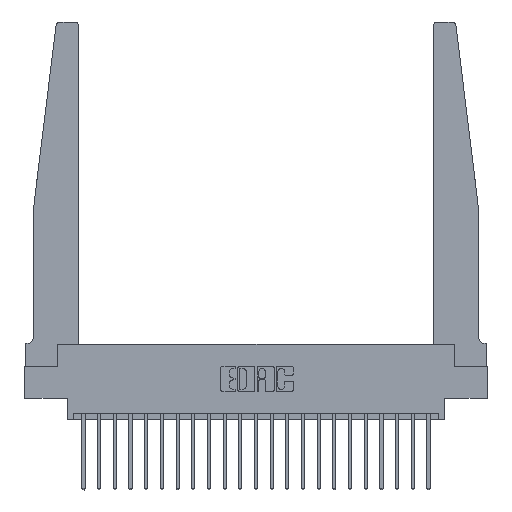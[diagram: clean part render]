
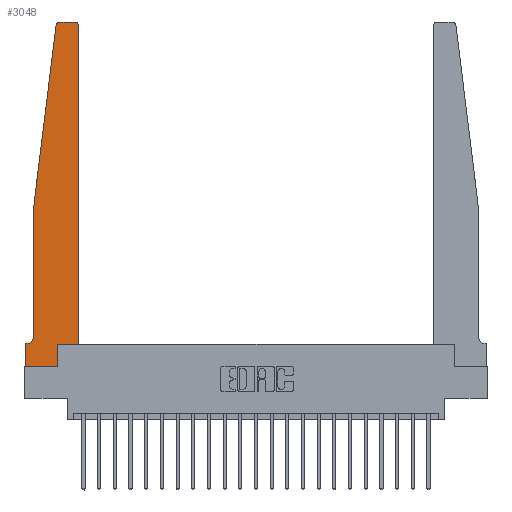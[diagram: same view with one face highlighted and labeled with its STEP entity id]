
A CAD part, top view. The second image highlights one B-rep face of the part: STEP entity #3048.
In plain terms, the highlighted planar face has unit normal (0, 0, 1).
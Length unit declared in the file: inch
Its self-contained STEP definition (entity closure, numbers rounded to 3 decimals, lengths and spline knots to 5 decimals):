
#40 = CARTESIAN_POINT ( 'NONE',  ( 0., 0.1875, 0.37 ) ) ;
#45 = CARTESIAN_POINT ( 'NONE',  ( 0., 0., 0.37 ) ) ;
#124 = EDGE_CURVE ( 'NONE', #2681, #18343, #1156, .T. ) ;
#596 = VECTOR ( 'NONE', #16283, 39.37008 ) ;
#807 = CARTESIAN_POINT ( 'NONE',  ( 0.425, 0.18, 0.37 ) ) ;
#1056 = CARTESIAN_POINT ( 'NONE',  ( 0.015, 0.2375, 0.37 ) ) ;
#1156 = LINE ( 'NONE', #21388, #596 ) ;
#1567 = AXIS2_PLACEMENT_3D ( 'NONE', #7672, #19767, #9418 ) ;
#1775 = CARTESIAN_POINT ( 'NONE',  ( 0.425, 0.18, 0.37 ) ) ;
#1826 = DIRECTION ( 'NONE',  ( 1., 0., 0. ) ) ;
#1832 = DIRECTION ( 'NONE',  ( 0., -1., 0. ) ) ;
#2221 = CARTESIAN_POINT ( 'NONE',  ( 0.24675, 2.72367, 0.37 ) ) ;
#2587 = VERTEX_POINT ( 'NONE', #7590 ) ;
#2681 = VERTEX_POINT ( 'NONE', #16542 ) ;
#2718 = LINE ( 'NONE', #1775, #20107 ) ;
#2743 = LINE ( 'NONE', #8662, #16095 ) ;
#2776 = VERTEX_POINT ( 'NONE', #20132 ) ;
#2807 = DIRECTION ( 'NONE',  ( -1., 0., 0. ) ) ;
#3048 = ADVANCED_FACE ( 'NONE', ( #13934 ), #20865, .T. ) ;
#3137 = LINE ( 'NONE', #6098, #7814 ) ;
#3323 = AXIS2_PLACEMENT_3D ( 'NONE', #40, #12265, #1826 ) ;
#3652 = EDGE_LOOP ( 'NONE', ( #15649, #20769, #12135, #21859, #3939, #18905, #20501, #7257, #21600, #13485, #5334, #9979 ) ) ;
#3723 = VERTEX_POINT ( 'NONE', #5247 ) ;
#3742 = CARTESIAN_POINT ( 'NONE',  ( 0.065, 1.25, 0.37 ) ) ;
#3843 = LINE ( 'NONE', #7886, #7979 ) ;
#3939 = ORIENTED_EDGE ( 'NONE', *, *, #8789, .T. ) ;
#4183 = EDGE_CURVE ( 'NONE', #18343, #2776, #2743, .T. ) ;
#4529 = CARTESIAN_POINT ( 'NONE',  ( 0.395, 2.75, 0.37 ) ) ;
#4591 = AXIS2_PLACEMENT_3D ( 'NONE', #1056, #13247, #2807 ) ;
#4999 = DIRECTION ( 'NONE',  ( 0., -1., 0. ) ) ;
#5247 = CARTESIAN_POINT ( 'NONE',  ( 0., 0.1875, 0.37 ) ) ;
#5334 = ORIENTED_EDGE ( 'NONE', *, *, #10177, .T. ) ;
#5709 = EDGE_CURVE ( 'NONE', #22224, #11923, #6277, .T. ) ;
#6098 = CARTESIAN_POINT ( 'NONE',  ( 0.065, 0.1875, 0.37 ) ) ;
#6116 = DIRECTION ( 'NONE',  ( 1., 0., 0. ) ) ;
#6268 = CARTESIAN_POINT ( 'NONE',  ( 0.27653, 2.75, 0.37 ) ) ;
#6277 = LINE ( 'NONE', #3742, #16024 ) ;
#7116 = LINE ( 'NONE', #45, #15779 ) ;
#7257 = ORIENTED_EDGE ( 'NONE', *, *, #124, .T. ) ;
#7590 = CARTESIAN_POINT ( 'NONE',  ( 0.425, 2.72, 0.37 ) ) ;
#7672 = CARTESIAN_POINT ( 'NONE',  ( 0.27653, 2.72, 0.37 ) ) ;
#7814 = VECTOR ( 'NONE', #14745, 39.37008 ) ;
#7886 = CARTESIAN_POINT ( 'NONE',  ( 0.25, 2.75, 0.37 ) ) ;
#7979 = VECTOR ( 'NONE', #9639, 39.37008 ) ;
#8292 = EDGE_CURVE ( 'NONE', #11923, #20949, #19123, .T. ) ;
#8516 = CARTESIAN_POINT ( 'NONE',  ( 0.065, 1.25, 0.37 ) ) ;
#8662 = CARTESIAN_POINT ( 'NONE',  ( 0.2605, 0.18, 0.37 ) ) ;
#8789 = EDGE_CURVE ( 'NONE', #20949, #18746, #19098, .T. ) ;
#8946 = EDGE_CURVE ( 'NONE', #2587, #12451, #20955, .T. ) ;
#9377 = VECTOR ( 'NONE', #4999, 39.37008 ) ;
#9418 = DIRECTION ( 'NONE',  ( 1., 0., 0. ) ) ;
#9639 = DIRECTION ( 'NONE',  ( -1., 0., 0. ) ) ;
#9979 = ORIENTED_EDGE ( 'NONE', *, *, #8946, .T. ) ;
#10177 = EDGE_CURVE ( 'NONE', #18912, #2587, #2718, .T. ) ;
#10218 = CARTESIAN_POINT ( 'NONE',  ( 0.395, 2.72, 0.37 ) ) ;
#10550 = CARTESIAN_POINT ( 'NONE',  ( 0.015, 0.1875, 0.37 ) ) ;
#11923 = VERTEX_POINT ( 'NONE', #8516 ) ;
#11967 = DIRECTION ( 'NONE',  ( 1., 0., 0. ) ) ;
#12135 = ORIENTED_EDGE ( 'NONE', *, *, #5709, .T. ) ;
#12227 = DIRECTION ( 'NONE',  ( 0., 1., 0. ) ) ;
#12265 = DIRECTION ( 'NONE',  ( 0., 0., 1. ) ) ;
#12451 = VERTEX_POINT ( 'NONE', #4529 ) ;
#12926 = EDGE_CURVE ( 'NONE', #2776, #18912, #21606, .T. ) ;
#13247 = DIRECTION ( 'NONE',  ( 0., 0., -1. ) ) ;
#13485 = ORIENTED_EDGE ( 'NONE', *, *, #12926, .T. ) ;
#13730 = EDGE_CURVE ( 'NONE', #18746, #3723, #3137, .T. ) ;
#13934 = FACE_OUTER_BOUND ( 'NONE', #3652, .T. ) ;
#14374 = EDGE_CURVE ( 'NONE', #21360, #22224, #19311, .T. ) ;
#14745 = DIRECTION ( 'NONE',  ( -1., 0., 0. ) ) ;
#14801 = EDGE_CURVE ( 'NONE', #3723, #2681, #7116, .T. ) ;
#15066 = AXIS2_PLACEMENT_3D ( 'NONE', #10218, #22307, #11967 ) ;
#15649 = ORIENTED_EDGE ( 'NONE', *, *, #20711, .T. ) ;
#15779 = VECTOR ( 'NONE', #1832, 39.37008 ) ;
#16024 = VECTOR ( 'NONE', #17665, 39.37008 ) ;
#16095 = VECTOR ( 'NONE', #19024, 39.37008 ) ;
#16161 = CARTESIAN_POINT ( 'NONE',  ( 0.425, 0.18, 0.37 ) ) ;
#16283 = DIRECTION ( 'NONE',  ( 1., 0., 0. ) ) ;
#16497 = VECTOR ( 'NONE', #6116, 39.37008 ) ;
#16542 = CARTESIAN_POINT ( 'NONE',  ( 0., 0., 0.37 ) ) ;
#17051 = CARTESIAN_POINT ( 'NONE',  ( 0.065, 0.2375, 0.37 ) ) ;
#17149 = CARTESIAN_POINT ( 'NONE',  ( 0.065, 1.25, 0.37 ) ) ;
#17665 = DIRECTION ( 'NONE',  ( -0.122, -0.992, 0. ) ) ;
#17777 = CARTESIAN_POINT ( 'NONE',  ( 0.2605, 0., 0.37 ) ) ;
#18343 = VERTEX_POINT ( 'NONE', #17777 ) ;
#18746 = VERTEX_POINT ( 'NONE', #10550 ) ;
#18905 = ORIENTED_EDGE ( 'NONE', *, *, #13730, .T. ) ;
#18912 = VERTEX_POINT ( 'NONE', #16161 ) ;
#19024 = DIRECTION ( 'NONE',  ( 0., 1., 0. ) ) ;
#19098 = CIRCLE ( 'NONE', #4591, 0.05 ) ;
#19123 = LINE ( 'NONE', #17149, #9377 ) ;
#19311 = CIRCLE ( 'NONE', #1567, 0.03 ) ;
#19767 = DIRECTION ( 'NONE',  ( 0., 0., 1. ) ) ;
#20107 = VECTOR ( 'NONE', #12227, 39.37008 ) ;
#20132 = CARTESIAN_POINT ( 'NONE',  ( 0.2605, 0.18, 0.37 ) ) ;
#20501 = ORIENTED_EDGE ( 'NONE', *, *, #14801, .T. ) ;
#20711 = EDGE_CURVE ( 'NONE', #12451, #21360, #3843, .T. ) ;
#20769 = ORIENTED_EDGE ( 'NONE', *, *, #14374, .T. ) ;
#20865 = PLANE ( 'NONE',  #3323 ) ;
#20949 = VERTEX_POINT ( 'NONE', #17051 ) ;
#20955 = CIRCLE ( 'NONE', #15066, 0.03 ) ;
#21360 = VERTEX_POINT ( 'NONE', #6268 ) ;
#21388 = CARTESIAN_POINT ( 'NONE',  ( 0., 0., 0.37 ) ) ;
#21600 = ORIENTED_EDGE ( 'NONE', *, *, #4183, .T. ) ;
#21606 = LINE ( 'NONE', #807, #16497 ) ;
#21859 = ORIENTED_EDGE ( 'NONE', *, *, #8292, .T. ) ;
#22224 = VERTEX_POINT ( 'NONE', #2221 ) ;
#22307 = DIRECTION ( 'NONE',  ( 0., 0., 1. ) ) ;
